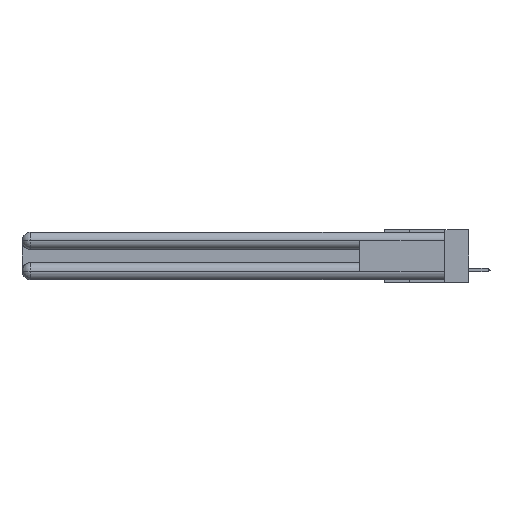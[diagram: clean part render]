
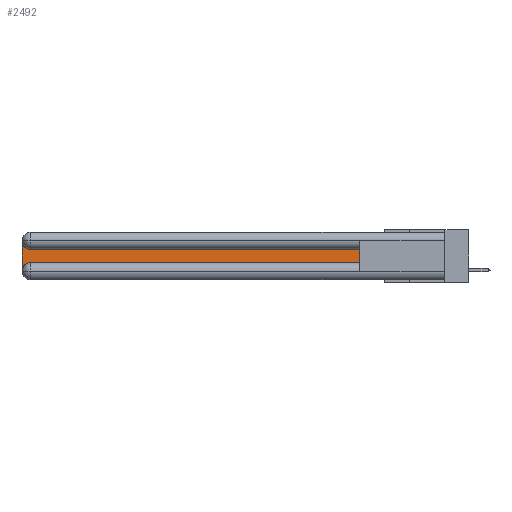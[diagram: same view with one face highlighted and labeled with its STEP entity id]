
A CAD part, left-side view. The second image highlights one B-rep face of the part: STEP entity #2492.
In plain terms, the highlighted planar face has unit normal (-1, 0, 0).
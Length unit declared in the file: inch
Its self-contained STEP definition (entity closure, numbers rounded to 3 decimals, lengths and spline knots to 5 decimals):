
#1159 = EDGE_CURVE ( 'NONE', #7753, #6326, #23191, .T. ) ;
#1662 = FACE_OUTER_BOUND ( 'NONE', #29641, .T. ) ;
#1812 = PLANE ( 'NONE',  #5205 ) ;
#1939 = ORIENTED_EDGE ( 'NONE', *, *, #13462, .T. ) ;
#2023 = CARTESIAN_POINT ( 'NONE',  ( 0.075, 0.6, -0.1225 ) ) ;
#2492 = ADVANCED_FACE ( 'NONE', ( #1662 ), #1812, .F. ) ;
#2543 = DIRECTION ( 'NONE',  ( 0., -1., 0. ) ) ;
#2938 = CARTESIAN_POINT ( 'NONE',  ( 0.075, 2.94, -0.1225 ) ) ;
#5205 = AXIS2_PLACEMENT_3D ( 'NONE', #19531, #9433, #9535 ) ;
#5251 = CARTESIAN_POINT ( 'NONE',  ( 0.075, 0.6, -0.2175 ) ) ;
#5483 = VECTOR ( 'NONE', #20447, 39.37008 ) ;
#6326 = VERTEX_POINT ( 'NONE', #31309 ) ;
#7582 = CARTESIAN_POINT ( 'NONE',  ( 0.075, 3., -0.2175 ) ) ;
#7753 = VERTEX_POINT ( 'NONE', #28152 ) ;
#8295 = ORIENTED_EDGE ( 'NONE', *, *, #1159, .T. ) ;
#9433 = DIRECTION ( 'NONE',  ( 1., 0., 0. ) ) ;
#9535 = DIRECTION ( 'NONE',  ( 0., 0., -1. ) ) ;
#9562 = CIRCLE ( 'NONE', #25757, 0.06 ) ;
#9679 = DIRECTION ( 'NONE',  ( 1., 0., 0. ) ) ;
#10138 = VERTEX_POINT ( 'NONE', #2938 ) ;
#10522 = CARTESIAN_POINT ( 'NONE',  ( 0.075, 0.6, -0.2175 ) ) ;
#11463 = VECTOR ( 'NONE', #2543, 39.37008 ) ;
#11633 = VECTOR ( 'NONE', #21300, 39.37008 ) ;
#12970 = EDGE_CURVE ( 'NONE', #27994, #16286, #27823, .T. ) ;
#13462 = EDGE_CURVE ( 'NONE', #10138, #32530, #9562, .T. ) ;
#15199 = CARTESIAN_POINT ( 'NONE',  ( 0.075, 3., -0.0625 ) ) ;
#16286 = VERTEX_POINT ( 'NONE', #2023 ) ;
#18765 = CARTESIAN_POINT ( 'NONE',  ( 0.075, 2.94, -0.0625 ) ) ;
#19325 = ORIENTED_EDGE ( 'NONE', *, *, #19657, .T. ) ;
#19531 = CARTESIAN_POINT ( 'NONE',  ( 0.075, 3., -0.1225 ) ) ;
#19657 = EDGE_CURVE ( 'NONE', #16286, #10138, #32231, .T. ) ;
#20447 = DIRECTION ( 'NONE',  ( 0., 0., -1. ) ) ;
#21300 = DIRECTION ( 'NONE',  ( 0., 1., 0. ) ) ;
#23191 = CIRCLE ( 'NONE', #28088, 0.06 ) ;
#24750 = DIRECTION ( 'NONE',  ( 0., 0., 1. ) ) ;
#24995 = CARTESIAN_POINT ( 'NONE',  ( 0.075, 2.94, -0.2775 ) ) ;
#25742 = LINE ( 'NONE', #5251, #11463 ) ;
#25757 = AXIS2_PLACEMENT_3D ( 'NONE', #18765, #28838, #29051 ) ;
#25866 = VECTOR ( 'NONE', #24750, 39.37008 ) ;
#26452 = ORIENTED_EDGE ( 'NONE', *, *, #28694, .T. ) ;
#27532 = DIRECTION ( 'NONE',  ( 0., 0., -1. ) ) ;
#27823 = LINE ( 'NONE', #31499, #25866 ) ;
#27853 = EDGE_CURVE ( 'NONE', #6326, #27994, #25742, .T. ) ;
#27993 = ORIENTED_EDGE ( 'NONE', *, *, #27853, .T. ) ;
#27994 = VERTEX_POINT ( 'NONE', #10522 ) ;
#28088 = AXIS2_PLACEMENT_3D ( 'NONE', #24995, #9679, #27532 ) ;
#28152 = CARTESIAN_POINT ( 'NONE',  ( 0.075, 3., -0.2775 ) ) ;
#28694 = EDGE_CURVE ( 'NONE', #32530, #7753, #30005, .T. ) ;
#28838 = DIRECTION ( 'NONE',  ( 1., 0., 0. ) ) ;
#28936 = CARTESIAN_POINT ( 'NONE',  ( 0.075, 0.6, -0.1225 ) ) ;
#29051 = DIRECTION ( 'NONE',  ( 0., 0., -1. ) ) ;
#29641 = EDGE_LOOP ( 'NONE', ( #19325, #1939, #26452, #8295, #27993, #29976 ) ) ;
#29976 = ORIENTED_EDGE ( 'NONE', *, *, #12970, .T. ) ;
#30005 = LINE ( 'NONE', #7582, #5483 ) ;
#31309 = CARTESIAN_POINT ( 'NONE',  ( 0.075, 2.94, -0.2175 ) ) ;
#31499 = CARTESIAN_POINT ( 'NONE',  ( 0.075, 0.6, -0.2175 ) ) ;
#32231 = LINE ( 'NONE', #28936, #11633 ) ;
#32530 = VERTEX_POINT ( 'NONE', #15199 ) ;
